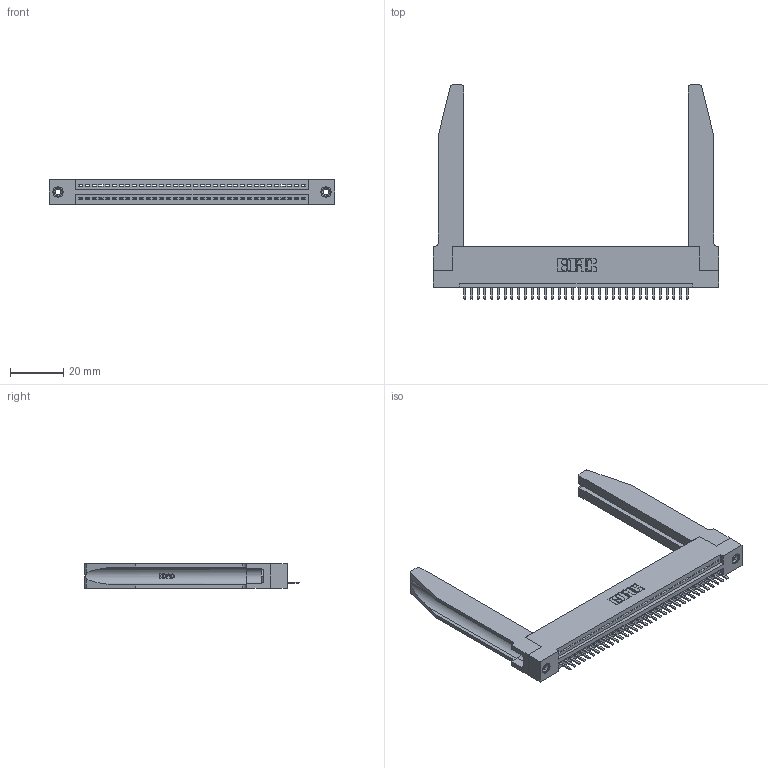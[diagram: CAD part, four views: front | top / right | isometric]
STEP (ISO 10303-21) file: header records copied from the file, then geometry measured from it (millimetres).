
FILE_DESCRIPTION (( 'STEP AP203' ), '1' );
FILE_NAME ('345-034-520-178.STEP', '2019-10-07T18:28:04', ( '' ), ( '' ), 'SwSTEP 2.0', 'SolidWorks 2016', '' );
FILE_SCHEMA (( 'CONFIG_CONTROL_DESIGN' ));
Length unit declared in the file: inch
Products named in the file (5): 345-034-520-178; 345 Part_Flush Mounting Lugs - 0.156 Dia-TH; 345-250-001_345-250-001-102; 345-292-001_345-293-120; 345-220-078_345-220-078
Assembly tree (39 placements, depth 2):
  345-034-520-178
    345 Part_Flush Mounting Lugs - 0.156 Dia-TH
    345-292-001_345-293-120  x34
    345-250-001_345-250-001-102  x2
    345-220-078_345-220-078  x2
Bounding box: 107.59 x 80.64 x 9.4 mm (x, y, z)
Volume: 17826.6 mm3; surface area: 19780.5 mm2
Topology: 39 solids, 39 shells, 2468 faces, 7205 edges, 4702 vertices
Faces by surface type: plane 1650, cylinder 766, bspline 36, cone 12, torus 4
Entity records: 31520 total; most frequent: CARTESIAN_POINT 6369, ORIENTED_EDGE 5222, DIRECTION 4569, EDGE_CURVE 2611, VECTOR 2245, LINE 2245, VERTEX_POINT 1732, AXIS2_PLACEMENT_3D 1162
